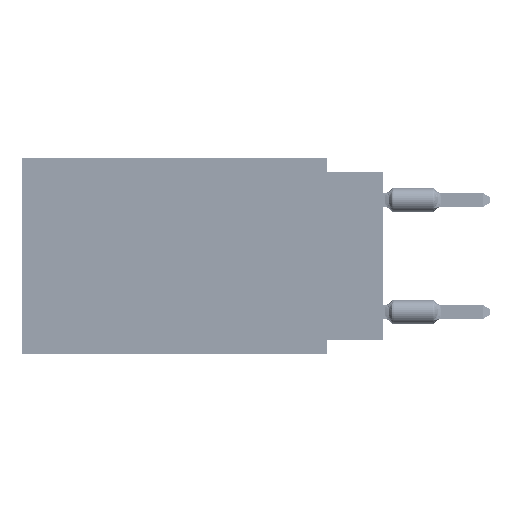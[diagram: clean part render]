
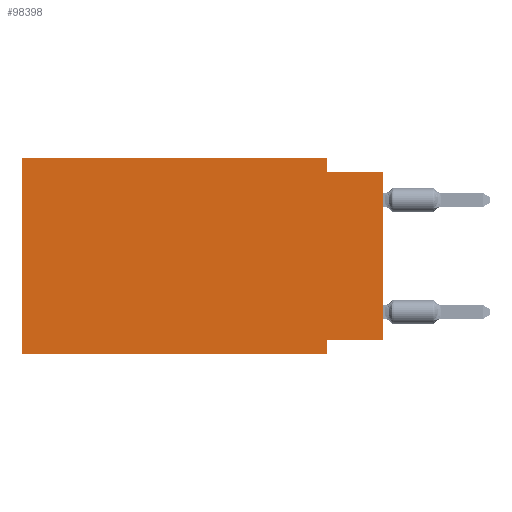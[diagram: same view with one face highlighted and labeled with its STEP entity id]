
A CAD part, left-side view. The second image highlights one B-rep face of the part: STEP entity #98398.
In plain terms, the highlighted planar face has unit normal (-1, 0, 0).
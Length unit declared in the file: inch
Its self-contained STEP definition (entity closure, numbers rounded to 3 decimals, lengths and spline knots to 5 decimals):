
#562 = CARTESIAN_POINT ( 'NONE',  ( 0., 0.645, 0. ) ) ;
#3137 = CARTESIAN_POINT ( 'NONE',  ( 0., 0., -0.325 ) ) ;
#3300 = CARTESIAN_POINT ( 'NONE',  ( 0., 0., -0.325 ) ) ;
#6096 = VECTOR ( 'NONE', #41771, 39.37008 ) ;
#6267 = LINE ( 'NONE', #48376, #21495 ) ;
#7333 = ORIENTED_EDGE ( 'NONE', *, *, #57880, .F. ) ;
#9586 = CARTESIAN_POINT ( 'NONE',  ( 0., 0.1, -0.35 ) ) ;
#13079 = LINE ( 'NONE', #47852, #27991 ) ;
#16210 = EDGE_CURVE ( 'NONE', #98243, #79363, #13079, .T. ) ;
#21495 = VECTOR ( 'NONE', #40507, 39.37008 ) ;
#21700 = VECTOR ( 'NONE', #102380, 39.37008 ) ;
#22921 = VERTEX_POINT ( 'NONE', #3300 ) ;
#24692 = DIRECTION ( 'NONE',  ( 1., 0., 0. ) ) ;
#24981 = CARTESIAN_POINT ( 'NONE',  ( 0., 0.1, 0. ) ) ;
#25925 = VERTEX_POINT ( 'NONE', #27587 ) ;
#26323 = ORIENTED_EDGE ( 'NONE', *, *, #30685, .F. ) ;
#26374 = FACE_OUTER_BOUND ( 'NONE', #31659, .T. ) ;
#26596 = CARTESIAN_POINT ( 'NONE',  ( 0., 0.645, 0. ) ) ;
#27587 = CARTESIAN_POINT ( 'NONE',  ( 0., 0., -0.025 ) ) ;
#27610 = ORIENTED_EDGE ( 'NONE', *, *, #29380, .F. ) ;
#27846 = DIRECTION ( 'NONE',  ( 0., 1., 0. ) ) ;
#27991 = VECTOR ( 'NONE', #47311, 39.37008 ) ;
#29380 = EDGE_CURVE ( 'NONE', #79363, #101244, #76596, .T. ) ;
#30685 = EDGE_CURVE ( 'NONE', #101244, #25925, #101239, .T. ) ;
#30988 = VERTEX_POINT ( 'NONE', #80978 ) ;
#31659 = EDGE_LOOP ( 'NONE', ( #59423, #26323, #27610, #43415, #102644, #101781, #7333, #85796 ) ) ;
#32434 = CARTESIAN_POINT ( 'NONE',  ( 0., 0.1, -0.025 ) ) ;
#33921 = CARTESIAN_POINT ( 'NONE',  ( 0., 0.645, -0.35 ) ) ;
#34805 = DIRECTION ( 'NONE',  ( 0., 0., -1. ) ) ;
#35459 = AXIS2_PLACEMENT_3D ( 'NONE', #562, #24692, #34805 ) ;
#35976 = DIRECTION ( 'NONE',  ( 0., 0., -1. ) ) ;
#40507 = DIRECTION ( 'NONE',  ( 0., 0., 1. ) ) ;
#40592 = EDGE_CURVE ( 'NONE', #30988, #73220, #110798, .T. ) ;
#41771 = DIRECTION ( 'NONE',  ( 0., -1., 0. ) ) ;
#42303 = EDGE_CURVE ( 'NONE', #22921, #25925, #6267, .T. ) ;
#43415 = ORIENTED_EDGE ( 'NONE', *, *, #16210, .F. ) ;
#47311 = DIRECTION ( 'NONE',  ( 0., -1., 0. ) ) ;
#47852 = CARTESIAN_POINT ( 'NONE',  ( 0., 0.645, 0. ) ) ;
#48376 = CARTESIAN_POINT ( 'NONE',  ( 0., 0., 0. ) ) ;
#49621 = DIRECTION ( 'NONE',  ( 0., 0., 1. ) ) ;
#57880 = EDGE_CURVE ( 'NONE', #105522, #73220, #86464, .T. ) ;
#59423 = ORIENTED_EDGE ( 'NONE', *, *, #42303, .T. ) ;
#61810 = EDGE_CURVE ( 'NONE', #30988, #98243, #75975, .T. ) ;
#70654 = VECTOR ( 'NONE', #35976, 39.37008 ) ;
#73220 = VERTEX_POINT ( 'NONE', #106551 ) ;
#74459 = CARTESIAN_POINT ( 'NONE',  ( 0., 0.1, 0. ) ) ;
#74795 = VECTOR ( 'NONE', #49621, 39.37008 ) ;
#75975 = LINE ( 'NONE', #26596, #74795 ) ;
#76596 = LINE ( 'NONE', #24981, #100772 ) ;
#79363 = VERTEX_POINT ( 'NONE', #74459 ) ;
#80809 = EDGE_CURVE ( 'NONE', #22921, #105522, #105828, .T. ) ;
#80978 = CARTESIAN_POINT ( 'NONE',  ( 0., 0.645, -0.35 ) ) ;
#85796 = ORIENTED_EDGE ( 'NONE', *, *, #80809, .F. ) ;
#86464 = LINE ( 'NONE', #9586, #70654 ) ;
#91490 = CARTESIAN_POINT ( 'NONE',  ( 0., 0.645, 0. ) ) ;
#94814 = PLANE ( 'NONE',  #35459 ) ;
#98243 = VERTEX_POINT ( 'NONE', #91490 ) ;
#98398 = ADVANCED_FACE ( 'NONE', ( #26374 ), #94814, .F. ) ;
#100772 = VECTOR ( 'NONE', #110284, 39.37008 ) ;
#101205 = VECTOR ( 'NONE', #27846, 39.37008 ) ;
#101239 = LINE ( 'NONE', #102373, #6096 ) ;
#101244 = VERTEX_POINT ( 'NONE', #32434 ) ;
#101781 = ORIENTED_EDGE ( 'NONE', *, *, #40592, .T. ) ;
#102373 = CARTESIAN_POINT ( 'NONE',  ( 0., 0., -0.025 ) ) ;
#102380 = DIRECTION ( 'NONE',  ( 0., -1., 0. ) ) ;
#102644 = ORIENTED_EDGE ( 'NONE', *, *, #61810, .F. ) ;
#105522 = VERTEX_POINT ( 'NONE', #110826 ) ;
#105828 = LINE ( 'NONE', #3137, #101205 ) ;
#106551 = CARTESIAN_POINT ( 'NONE',  ( 0., 0.1, -0.35 ) ) ;
#110284 = DIRECTION ( 'NONE',  ( 0., 0., -1. ) ) ;
#110798 = LINE ( 'NONE', #33921, #21700 ) ;
#110826 = CARTESIAN_POINT ( 'NONE',  ( 0., 0.1, -0.325 ) ) ;
